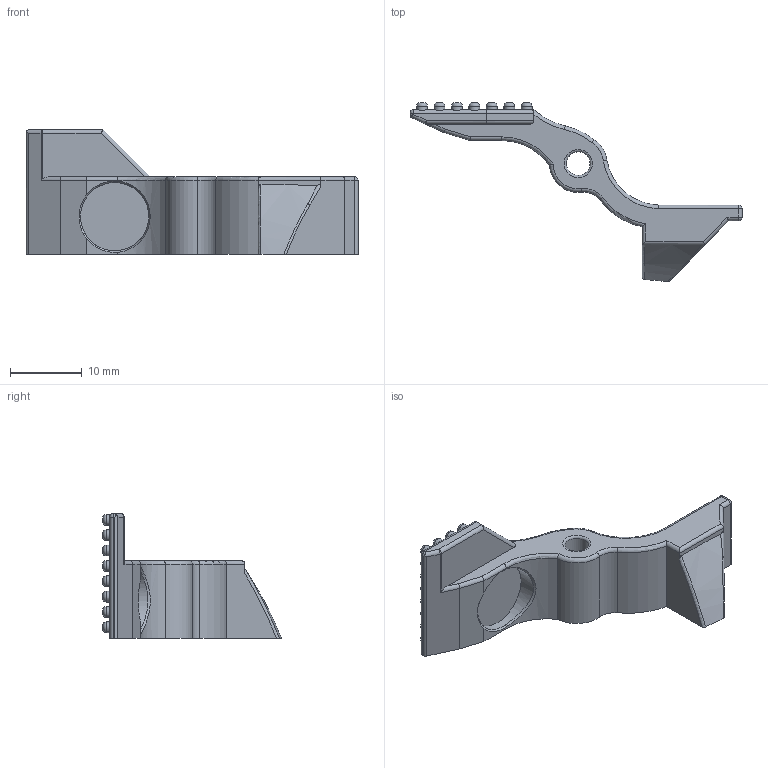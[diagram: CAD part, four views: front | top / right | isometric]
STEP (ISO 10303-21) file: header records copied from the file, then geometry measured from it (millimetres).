
FILE_DESCRIPTION(/* description */ (''),/* implementation_level */ '2;1');
FILE_NAME(/* name */ 'AWCY_HOLSTER_RELEASEV3.step',/* time_stamp */ '2020-09-01T21:05:14-07:00',/* author */ (''),/* organization */ (''),/* preprocessor_version */ 'ST-DEVELOPER v18.1',/* originating_system */ 'Autodesk Translation Framework v9.3.0.1241',/* authorisation */ '');
FILE_SCHEMA (('AUTOMOTIVE_DESIGN { 1 0 10303 214 3 1 1 }'));
Length unit declared in the file: millimetre
Products named in the file (1): AWCY_DSGLOCKS_HOLSTER_V3
Bounding box: 46.16 x 24.87 x 17.36 mm (x, y, z)
Volume: 2673.4 mm3; surface area: 2197.6 mm2
Topology: 1 solids, 1 shells, 224 faces, 496 edges, 318 vertices
Faces by surface type: cylinder 82, plane 69, bspline 57, torus 10, sphere 4, cone 2
Full cylindrical faces by diameter (mm): 1.5 x50, 3.3 x1, 9.5 x1
Entity records: 7867 total; most frequent: CARTESIAN_POINT 2822, DIRECTION 1136, ORIENTED_EDGE 990, AXIS2_PLACEMENT_3D 501, EDGE_CURVE 495, VERTEX_POINT 318, CIRCLE 312, EDGE_LOOP 271
